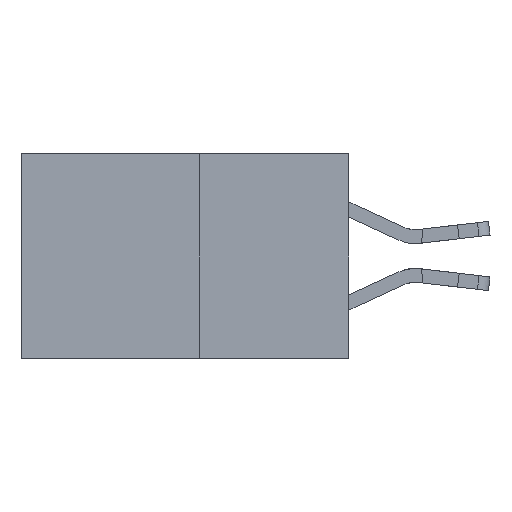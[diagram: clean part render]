
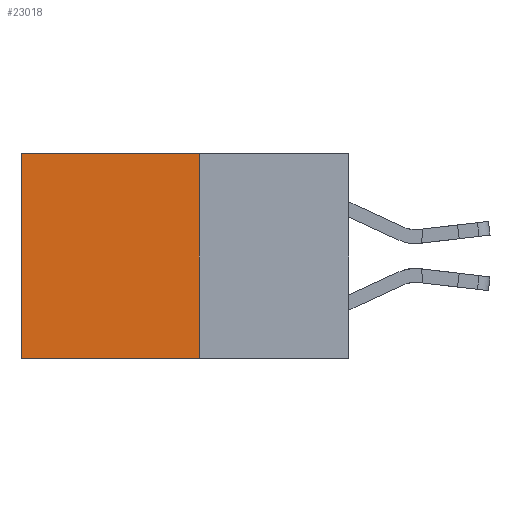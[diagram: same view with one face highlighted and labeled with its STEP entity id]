
A CAD part, left-side view. The second image highlights one B-rep face of the part: STEP entity #23018.
In plain terms, the highlighted planar face has unit normal (-1, 0, 0).
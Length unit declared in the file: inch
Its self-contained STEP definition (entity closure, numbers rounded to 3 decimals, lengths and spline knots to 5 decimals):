
#956 = DIRECTION ( 'NONE',  ( 0., 0., -1. ) ) ;
#1199 = CARTESIAN_POINT ( 'NONE',  ( 0.277, 0.27, -0.37 ) ) ;
#2197 = ORIENTED_EDGE ( 'NONE', *, *, #4469, .F. ) ;
#2262 = VERTEX_POINT ( 'NONE', #10821 ) ;
#2683 = LINE ( 'NONE', #4270, #13632 ) ;
#3272 = VECTOR ( 'NONE', #4722, 39.37008 ) ;
#3591 = DIRECTION ( 'NONE',  ( 0., 1., 0. ) ) ;
#4270 = CARTESIAN_POINT ( 'NONE',  ( 0.277, 0.27, -0.37 ) ) ;
#4469 = EDGE_CURVE ( 'NONE', #28433, #14235, #2683, .T. ) ;
#4722 = DIRECTION ( 'NONE',  ( 0., 0., -1. ) ) ;
#5682 = CARTESIAN_POINT ( 'NONE',  ( 0.277, 0.59, -0.37 ) ) ;
#5909 = VECTOR ( 'NONE', #7181, 39.37008 ) ;
#7181 = DIRECTION ( 'NONE',  ( 0., 1., 0. ) ) ;
#7197 = LINE ( 'NONE', #22554, #13381 ) ;
#8809 = DIRECTION ( 'NONE',  ( 0., 0., -1. ) ) ;
#8851 = EDGE_CURVE ( 'NONE', #2262, #28433, #7197, .T. ) ;
#10291 = PLANE ( 'NONE',  #27099 ) ;
#10821 = CARTESIAN_POINT ( 'NONE',  ( 0.277, 0.27, 0. ) ) ;
#13003 = ORIENTED_EDGE ( 'NONE', *, *, #18178, .T. ) ;
#13381 = VECTOR ( 'NONE', #8809, 39.37008 ) ;
#13632 = VECTOR ( 'NONE', #3591, 39.37008 ) ;
#13761 = VERTEX_POINT ( 'NONE', #18073 ) ;
#14235 = VERTEX_POINT ( 'NONE', #5682 ) ;
#14930 = DIRECTION ( 'NONE',  ( 1., 0., 0. ) ) ;
#16273 = EDGE_CURVE ( 'NONE', #2262, #13761, #24282, .T. ) ;
#16890 = EDGE_LOOP ( 'NONE', ( #13003, #2197, #21120, #25313 ) ) ;
#18073 = CARTESIAN_POINT ( 'NONE',  ( 0.277, 0.59, 0. ) ) ;
#18178 = EDGE_CURVE ( 'NONE', #13761, #14235, #27059, .T. ) ;
#18594 = CARTESIAN_POINT ( 'NONE',  ( 0.277, 0.59, -0.37 ) ) ;
#21120 = ORIENTED_EDGE ( 'NONE', *, *, #8851, .F. ) ;
#22554 = CARTESIAN_POINT ( 'NONE',  ( 0.277, 0.27, -0.37 ) ) ;
#23018 = ADVANCED_FACE ( 'NONE', ( #23488 ), #10291, .F. ) ;
#23271 = CARTESIAN_POINT ( 'NONE',  ( 0.277, 0.27, 0. ) ) ;
#23488 = FACE_OUTER_BOUND ( 'NONE', #16890, .T. ) ;
#24282 = LINE ( 'NONE', #23271, #5909 ) ;
#25313 = ORIENTED_EDGE ( 'NONE', *, *, #16273, .T. ) ;
#27059 = LINE ( 'NONE', #18594, #3272 ) ;
#27099 = AXIS2_PLACEMENT_3D ( 'NONE', #28572, #14930, #956 ) ;
#28433 = VERTEX_POINT ( 'NONE', #1199 ) ;
#28572 = CARTESIAN_POINT ( 'NONE',  ( 0.277, 0.27, -0.37 ) ) ;
